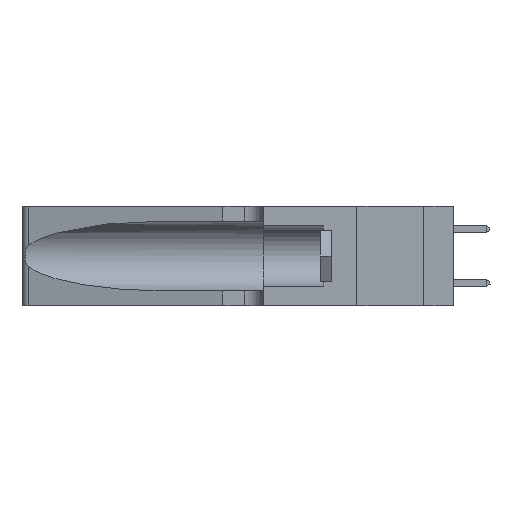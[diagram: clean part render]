
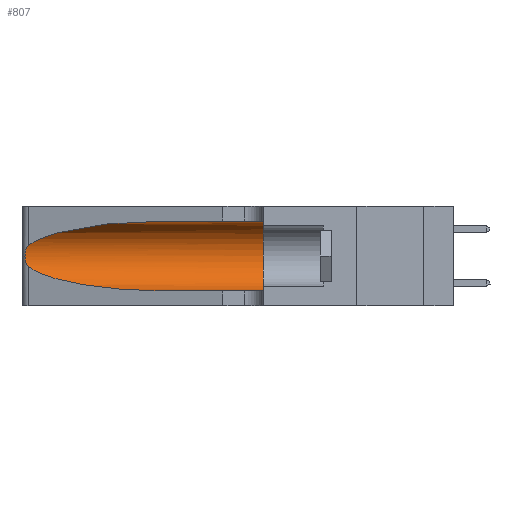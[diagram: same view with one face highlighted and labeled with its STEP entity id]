
A CAD part, left-side view. The second image highlights one B-rep face of the part: STEP entity #807.
In plain terms, the highlighted cylindrical face has radius 3.308 mm (diameter 6.617 mm), a partial arc.
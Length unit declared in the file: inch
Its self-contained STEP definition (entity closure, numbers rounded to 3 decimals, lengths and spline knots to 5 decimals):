
#34 = CARTESIAN_POINT ( 'NONE',  ( 0.1305, 0.72297, 0.05475 ) ) ;
#188 = CARTESIAN_POINT ( 'NONE',  ( 0.1305, 1.61858, 0.31525 ) ) ;
#380 = EDGE_CURVE ( 'NONE', #28341, #22212, #2896, .T. ) ;
#619 = CARTESIAN_POINT ( 'NONE',  ( 0.25487, 1.22718, 0.22369 ) ) ;
#715 = CARTESIAN_POINT ( 'NONE',  ( 0.25555, 1.22994, 0.2215 ) ) ;
#807 = ADVANCED_FACE ( 'NONE', ( #11602 ), #15737, .F. ) ;
#820 = CARTESIAN_POINT ( 'NONE',  ( 0.25854, 1.2359, 0.20912 ) ) ;
#1557 = DIRECTION ( 'NONE',  ( 0., 1., 0. ) ) ;
#2896 =( BOUNDED_CURVE ( )  B_SPLINE_CURVE ( 3, ( #21276, #28730, #23677, #34 ),
 .UNSPECIFIED., .F., .F. ) 
 B_SPLINE_CURVE_WITH_KNOTS ( ( 4, 4 ),
 ( 3.44316, 4.71239 ),
 .UNSPECIFIED. ) 
 CURVE ( )  GEOMETRIC_REPRESENTATION_ITEM ( )  RATIONAL_B_SPLINE_CURVE ( ( 1., 0.87, 0.87, 1. ) ) 
 REPRESENTATION_ITEM ( '' )  );
#3132 = CARTESIAN_POINT ( 'NONE',  ( 0.25487, 1.22718, 0.14631 ) ) ;
#3280 = CARTESIAN_POINT ( 'NONE',  ( 0.26017, 1.23833, 0.17102 ) ) ;
#3727 = VERTEX_POINT ( 'NONE', #33794 ) ;
#6013 = ORIENTED_EDGE ( 'NONE', *, *, #11437, .T. ) ;
#6181 = CARTESIAN_POINT ( 'NONE',  ( 0.25639, 1.23184, 0.21858 ) ) ;
#6538 = CARTESIAN_POINT ( 'NONE',  ( 0.1305, 0.72297, 0.31525 ) ) ;
#6631 = LINE ( 'NONE', #188, #18123 ) ;
#8151 = DIRECTION ( 'NONE',  ( 0., 0., -1. ) ) ;
#8307 = EDGE_LOOP ( 'NONE', ( #6013, #13443, #13993, #15301, #22046, #29948 ) ) ;
#8478 = DIRECTION ( 'NONE',  ( 0., -1., 0. ) ) ;
#8637 = CARTESIAN_POINT ( 'NONE',  ( 0.25856, 1.23593, 0.16098 ) ) ;
#8660 = CARTESIAN_POINT ( 'NONE',  ( 0.2373, 1.15595, 0.28018 ) ) ;
#9350 = CIRCLE ( 'NONE', #22564, 0.13025 ) ;
#9676 = EDGE_CURVE ( 'NONE', #14841, #3727, #9350, .T. ) ;
#10763 = DIRECTION ( 'NONE',  ( 0., -1., 0. ) ) ;
#11072 = LINE ( 'NONE', #13037, #11448 ) ;
#11355 = CARTESIAN_POINT ( 'NONE',  ( 0.26018, 1.23835, 0.19895 ) ) ;
#11437 = EDGE_CURVE ( 'NONE', #15968, #33155, #14000, .T. ) ;
#11448 = VECTOR ( 'NONE', #8478, 39.37008 ) ;
#11564 = CARTESIAN_POINT ( 'NONE',  ( 0.25639, 1.23186, 0.15144 ) ) ;
#11602 = FACE_OUTER_BOUND ( 'NONE', #8307, .T. ) ;
#13037 = CARTESIAN_POINT ( 'NONE',  ( 0.1305, 1.61858, 0.05475 ) ) ;
#13066 = DIRECTION ( 'NONE',  ( 0., -1., 0. ) ) ;
#13443 = ORIENTED_EDGE ( 'NONE', *, *, #24000, .T. ) ;
#13849 = CARTESIAN_POINT ( 'NONE',  ( 0.1305, 0.72297, 0.31525 ) ) ;
#13993 = ORIENTED_EDGE ( 'NONE', *, *, #380, .T. ) ;
#14000 =( BOUNDED_CURVE ( )  B_SPLINE_CURVE ( 3, ( #13849, #24426, #8660, #619 ),
 .UNSPECIFIED., .F., .F. ) 
 B_SPLINE_CURVE_WITH_KNOTS ( ( 4, 4 ),
 ( 1.5708, 2.84003 ),
 .UNSPECIFIED. ) 
 CURVE ( )  GEOMETRIC_REPRESENTATION_ITEM ( )  RATIONAL_B_SPLINE_CURVE ( ( 1., 0.87, 0.87, 1. ) ) 
 REPRESENTATION_ITEM ( '' )  );
#14164 = CARTESIAN_POINT ( 'NONE',  ( 0.25487, 1.22718, 0.14631 ) ) ;
#14841 = VERTEX_POINT ( 'NONE', #23130 ) ;
#15301 = ORIENTED_EDGE ( 'NONE', *, *, #22254, .T. ) ;
#15737 = CYLINDRICAL_SURFACE ( 'NONE', #19040, 0.13025 ) ;
#15968 = VERTEX_POINT ( 'NONE', #6538 ) ;
#16465 = CARTESIAN_POINT ( 'NONE',  ( 0.25487, 1.22718, 0.22369 ) ) ;
#18123 = VECTOR ( 'NONE', #13066, 39.37008 ) ;
#19028 = CARTESIAN_POINT ( 'NONE',  ( 0.26075, 1.23896, 0.19203 ) ) ;
#19040 = AXIS2_PLACEMENT_3D ( 'NONE', #26456, #10763, #8151 ) ;
#19965 = DIRECTION ( 'NONE',  ( 0., 0., 1. ) ) ;
#20168 = CARTESIAN_POINT ( 'NONE',  ( 0.1305, 0.72297, 0.05475 ) ) ;
#21276 = CARTESIAN_POINT ( 'NONE',  ( 0.25487, 1.22718, 0.14631 ) ) ;
#22046 = ORIENTED_EDGE ( 'NONE', *, *, #9676, .F. ) ;
#22212 = VERTEX_POINT ( 'NONE', #20168 ) ;
#22254 = EDGE_CURVE ( 'NONE', #22212, #3727, #11072, .T. ) ;
#22564 = AXIS2_PLACEMENT_3D ( 'NONE', #33157, #1557, #19965 ) ;
#22718 = B_SPLINE_CURVE_WITH_KNOTS ( 'NONE', 3,
 ( #16465, #715, #6181, #27250, #820, #11355, #19028, #29693, #3280, #8637, #26931, #11564, #29926, #14164 ),
 .UNSPECIFIED., .F., .F.,
 ( 4, 2, 2, 2, 2, 2, 4 ),
 ( 0., 0.00027, 0.00053, 0.00107, 0.0016, 0.00187, 0.00214 ),
 .UNSPECIFIED. ) ;
#23130 = CARTESIAN_POINT ( 'NONE',  ( 0.1305, 0.35, 0.31525 ) ) ;
#23677 = CARTESIAN_POINT ( 'NONE',  ( 0.18966, 0.96281, 0.05475 ) ) ;
#24000 = EDGE_CURVE ( 'NONE', #33155, #28341, #22718, .T. ) ;
#24426 = CARTESIAN_POINT ( 'NONE',  ( 0.18966, 0.96281, 0.31525 ) ) ;
#26456 = CARTESIAN_POINT ( 'NONE',  ( 0.1305, 1.61858, 0.185 ) ) ;
#26524 = EDGE_CURVE ( 'NONE', #15968, #14841, #6631, .T. ) ;
#26931 = CARTESIAN_POINT ( 'NONE',  ( 0.25789, 1.23486, 0.15765 ) ) ;
#27250 = CARTESIAN_POINT ( 'NONE',  ( 0.25787, 1.23484, 0.2124 ) ) ;
#28341 = VERTEX_POINT ( 'NONE', #3132 ) ;
#28385 = CARTESIAN_POINT ( 'NONE',  ( 0.25487, 1.22718, 0.22369 ) ) ;
#28730 = CARTESIAN_POINT ( 'NONE',  ( 0.2373, 1.15595, 0.08982 ) ) ;
#29693 = CARTESIAN_POINT ( 'NONE',  ( 0.26075, 1.23896, 0.178 ) ) ;
#29926 = CARTESIAN_POINT ( 'NONE',  ( 0.25555, 1.22993, 0.14849 ) ) ;
#29948 = ORIENTED_EDGE ( 'NONE', *, *, #26524, .F. ) ;
#33155 = VERTEX_POINT ( 'NONE', #28385 ) ;
#33157 = CARTESIAN_POINT ( 'NONE',  ( 0.1305, 0.35, 0.185 ) ) ;
#33794 = CARTESIAN_POINT ( 'NONE',  ( 0.1305, 0.35, 0.05475 ) ) ;
